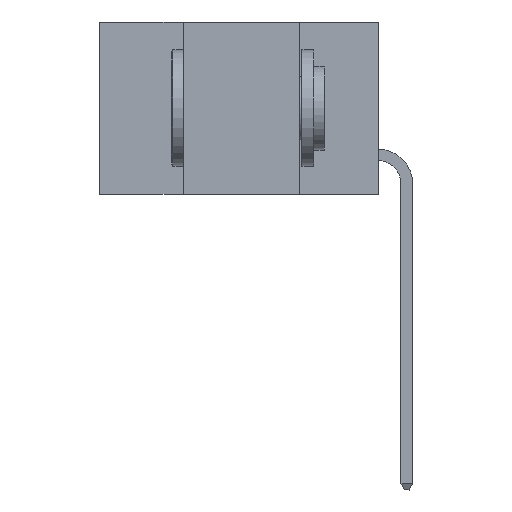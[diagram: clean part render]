
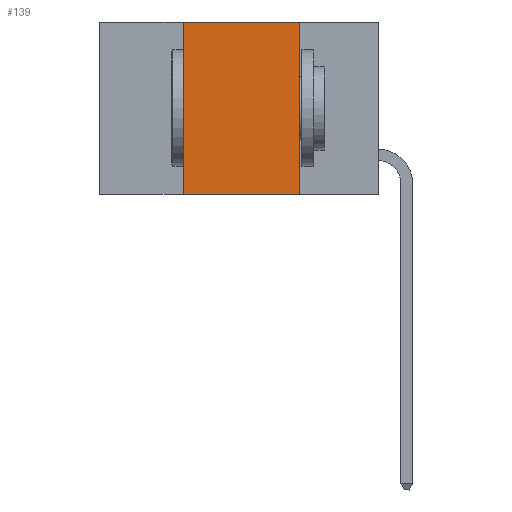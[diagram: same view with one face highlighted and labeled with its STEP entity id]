
A CAD part, left-side view. The second image highlights one B-rep face of the part: STEP entity #139.
In plain terms, the highlighted planar face has unit normal (-1, 0, 0).
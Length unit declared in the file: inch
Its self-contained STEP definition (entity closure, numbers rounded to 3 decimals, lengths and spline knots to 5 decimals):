
#139 = ADVANCED_FACE ( 'NONE', ( #17278 ), #9689, .F. ) ;
#824 = DIRECTION ( 'NONE',  ( 0., 0., -1. ) ) ;
#1022 = DIRECTION ( 'NONE',  ( 1., 0., 0. ) ) ;
#2817 = LINE ( 'NONE', #9802, #10040 ) ;
#3247 = VECTOR ( 'NONE', #3719, 39.37008 ) ;
#3389 = VECTOR ( 'NONE', #12442, 39.37008 ) ;
#3527 = LINE ( 'NONE', #14339, #7329 ) ;
#3719 = DIRECTION ( 'NONE',  ( 0., -1., 0. ) ) ;
#4158 = EDGE_CURVE ( 'NONE', #7195, #18410, #2817, .T. ) ;
#7195 = VERTEX_POINT ( 'NONE', #15356 ) ;
#7320 = AXIS2_PLACEMENT_3D ( 'NONE', #13660, #1022, #824 ) ;
#7329 = VECTOR ( 'NONE', #15343, 39.37008 ) ;
#7560 = EDGE_CURVE ( 'NONE', #7777, #18410, #18070, .T. ) ;
#7777 = VERTEX_POINT ( 'NONE', #12465 ) ;
#7972 = EDGE_LOOP ( 'NONE', ( #8558, #8812, #9449, #17024 ) ) ;
#8558 = ORIENTED_EDGE ( 'NONE', *, *, #7560, .F. ) ;
#8812 = ORIENTED_EDGE ( 'NONE', *, *, #14859, .F. ) ;
#9449 = ORIENTED_EDGE ( 'NONE', *, *, #9954, .F. ) ;
#9549 = LINE ( 'NONE', #12349, #3247 ) ;
#9689 = PLANE ( 'NONE',  #7320 ) ;
#9802 = CARTESIAN_POINT ( 'NONE',  ( 0., 0.6, -0.37 ) ) ;
#9954 = EDGE_CURVE ( 'NONE', #7195, #18380, #3527, .T. ) ;
#10040 = VECTOR ( 'NONE', #14546, 39.37008 ) ;
#12349 = CARTESIAN_POINT ( 'NONE',  ( 0., 0.6, 0. ) ) ;
#12442 = DIRECTION ( 'NONE',  ( 0., 0., -1. ) ) ;
#12465 = CARTESIAN_POINT ( 'NONE',  ( 0., 0.17, 0. ) ) ;
#12787 = CARTESIAN_POINT ( 'NONE',  ( 0., 0.17, 0. ) ) ;
#13660 = CARTESIAN_POINT ( 'NONE',  ( 0., 0.6, 0. ) ) ;
#14339 = CARTESIAN_POINT ( 'NONE',  ( 0., 0.42, 0. ) ) ;
#14546 = DIRECTION ( 'NONE',  ( 0., -1., 0. ) ) ;
#14859 = EDGE_CURVE ( 'NONE', #18380, #7777, #9549, .T. ) ;
#15343 = DIRECTION ( 'NONE',  ( 0., 0., 1. ) ) ;
#15356 = CARTESIAN_POINT ( 'NONE',  ( 0., 0.42, -0.37 ) ) ;
#16214 = CARTESIAN_POINT ( 'NONE',  ( 0., 0.17, -0.37 ) ) ;
#17024 = ORIENTED_EDGE ( 'NONE', *, *, #4158, .T. ) ;
#17278 = FACE_OUTER_BOUND ( 'NONE', #7972, .T. ) ;
#17542 = CARTESIAN_POINT ( 'NONE',  ( 0., 0.42, 0. ) ) ;
#18070 = LINE ( 'NONE', #12787, #3389 ) ;
#18380 = VERTEX_POINT ( 'NONE', #17542 ) ;
#18410 = VERTEX_POINT ( 'NONE', #16214 ) ;
